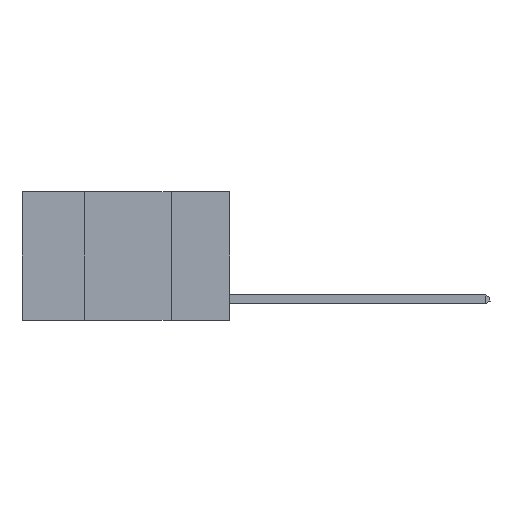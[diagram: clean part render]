
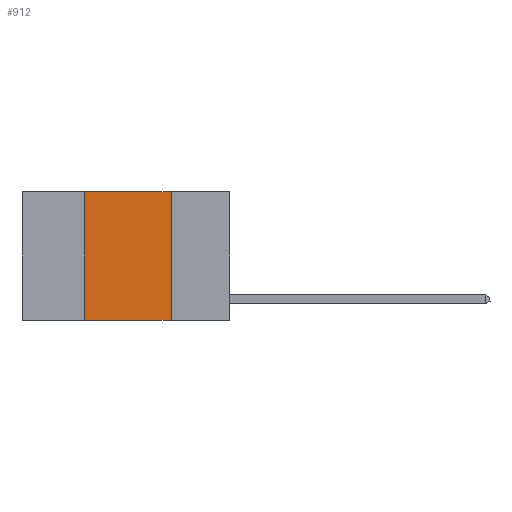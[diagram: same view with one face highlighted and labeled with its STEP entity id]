
A CAD part, left-side view. The second image highlights one B-rep face of the part: STEP entity #912.
In plain terms, the highlighted planar face has unit normal (-1, 0, 0).
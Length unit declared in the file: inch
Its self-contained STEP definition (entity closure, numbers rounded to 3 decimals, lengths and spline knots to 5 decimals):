
#503 = VERTEX_POINT ( 'NONE', #10407 ) ;
#912 = ADVANCED_FACE ( 'NONE', ( #12940 ), #12998, .F. ) ;
#1195 = EDGE_CURVE ( 'NONE', #503, #3126, #9218, .T. ) ;
#1794 = LINE ( 'NONE', #6017, #11764 ) ;
#1917 = CARTESIAN_POINT ( 'NONE',  ( 0., 0.17, 0. ) ) ;
#2131 = ORIENTED_EDGE ( 'NONE', *, *, #1195, .F. ) ;
#2370 = CARTESIAN_POINT ( 'NONE',  ( 0., 0.6, -0.37 ) ) ;
#2425 = CARTESIAN_POINT ( 'NONE',  ( 0., 0.6, 0. ) ) ;
#2982 = CARTESIAN_POINT ( 'NONE',  ( 0., 0.42, 0. ) ) ;
#3126 = VERTEX_POINT ( 'NONE', #5392 ) ;
#3590 = EDGE_CURVE ( 'NONE', #11081, #11615, #11682, .T. ) ;
#3865 = VECTOR ( 'NONE', #8041, 39.37008 ) ;
#3925 = VECTOR ( 'NONE', #10523, 39.37008 ) ;
#4902 = VECTOR ( 'NONE', #11315, 39.37008 ) ;
#5392 = CARTESIAN_POINT ( 'NONE',  ( 0., 0.42, 0. ) ) ;
#5696 = ORIENTED_EDGE ( 'NONE', *, *, #10005, .T. ) ;
#6017 = CARTESIAN_POINT ( 'NONE',  ( 0., 0.6, 0. ) ) ;
#6071 = DIRECTION ( 'NONE',  ( 0., -1., 0. ) ) ;
#7228 = LINE ( 'NONE', #2370, #4902 ) ;
#8041 = DIRECTION ( 'NONE',  ( 0., 0., -1. ) ) ;
#9218 = LINE ( 'NONE', #2982, #3925 ) ;
#9788 = CARTESIAN_POINT ( 'NONE',  ( 0., 0.17, -0.37 ) ) ;
#9959 = DIRECTION ( 'NONE',  ( 1., 0., 0. ) ) ;
#10005 = EDGE_CURVE ( 'NONE', #503, #11615, #7228, .T. ) ;
#10407 = CARTESIAN_POINT ( 'NONE',  ( 0., 0.42, -0.37 ) ) ;
#10494 = EDGE_CURVE ( 'NONE', #3126, #11081, #1794, .T. ) ;
#10523 = DIRECTION ( 'NONE',  ( 0., 0., 1. ) ) ;
#10590 = EDGE_LOOP ( 'NONE', ( #11512, #11888, #2131, #5696 ) ) ;
#11081 = VERTEX_POINT ( 'NONE', #12907 ) ;
#11315 = DIRECTION ( 'NONE',  ( 0., -1., 0. ) ) ;
#11512 = ORIENTED_EDGE ( 'NONE', *, *, #3590, .F. ) ;
#11615 = VERTEX_POINT ( 'NONE', #9788 ) ;
#11682 = LINE ( 'NONE', #1917, #3865 ) ;
#11764 = VECTOR ( 'NONE', #6071, 39.37008 ) ;
#11888 = ORIENTED_EDGE ( 'NONE', *, *, #10494, .F. ) ;
#12754 = AXIS2_PLACEMENT_3D ( 'NONE', #2425, #9959, #12955 ) ;
#12907 = CARTESIAN_POINT ( 'NONE',  ( 0., 0.17, 0. ) ) ;
#12940 = FACE_OUTER_BOUND ( 'NONE', #10590, .T. ) ;
#12955 = DIRECTION ( 'NONE',  ( 0., 0., -1. ) ) ;
#12998 = PLANE ( 'NONE',  #12754 ) ;
